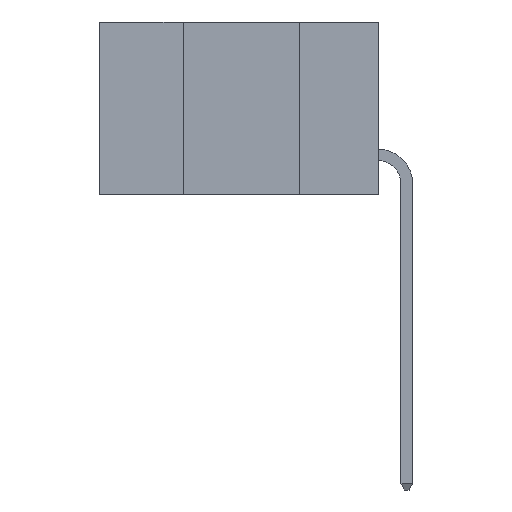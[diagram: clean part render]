
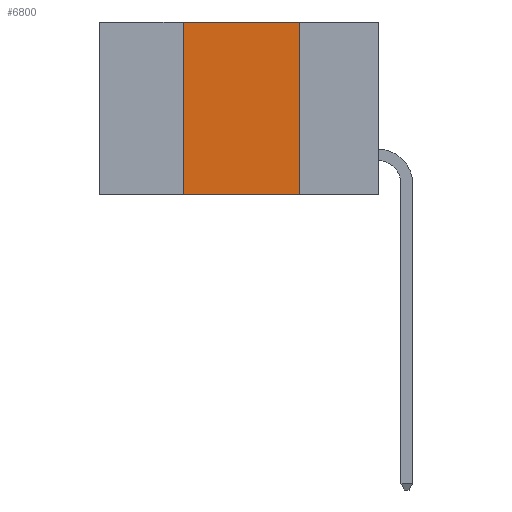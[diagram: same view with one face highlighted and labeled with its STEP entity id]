
A CAD part, left-side view. The second image highlights one B-rep face of the part: STEP entity #6800.
In plain terms, the highlighted planar face has unit normal (-1, 0, 0).
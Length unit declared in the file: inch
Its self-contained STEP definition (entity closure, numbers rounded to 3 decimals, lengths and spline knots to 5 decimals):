
#196 = LINE ( 'NONE', #5442, #4242 ) ;
#458 = CARTESIAN_POINT ( 'NONE',  ( 0., 0.6, -0.37 ) ) ;
#465 = CARTESIAN_POINT ( 'NONE',  ( 0., 0.42, -0.37 ) ) ;
#785 = CARTESIAN_POINT ( 'NONE',  ( 0., 0.17, -0.37 ) ) ;
#815 = EDGE_CURVE ( 'NONE', #5979, #6418, #4094, .T. ) ;
#880 = DIRECTION ( 'NONE',  ( 0., 0., -1. ) ) ;
#1025 = ORIENTED_EDGE ( 'NONE', *, *, #815, .T. ) ;
#1247 = DIRECTION ( 'NONE',  ( 0., -1., 0. ) ) ;
#1841 = VECTOR ( 'NONE', #7947, 39.37008 ) ;
#2918 = VERTEX_POINT ( 'NONE', #10349 ) ;
#3309 = LINE ( 'NONE', #8675, #5537 ) ;
#3411 = PLANE ( 'NONE',  #8020 ) ;
#3537 = VECTOR ( 'NONE', #880, 39.37008 ) ;
#3877 = EDGE_LOOP ( 'NONE', ( #5787, #9614, #7623, #1025 ) ) ;
#3914 = EDGE_CURVE ( 'NONE', #2918, #6418, #9583, .T. ) ;
#4094 = LINE ( 'NONE', #458, #1841 ) ;
#4242 = VECTOR ( 'NONE', #1247, 39.37008 ) ;
#4587 = CARTESIAN_POINT ( 'NONE',  ( 0., 0.42, 0. ) ) ;
#5096 = DIRECTION ( 'NONE',  ( 0., 0., -1. ) ) ;
#5289 = FACE_OUTER_BOUND ( 'NONE', #3877, .T. ) ;
#5442 = CARTESIAN_POINT ( 'NONE',  ( 0., 0.6, 0. ) ) ;
#5537 = VECTOR ( 'NONE', #9421, 39.37008 ) ;
#5787 = ORIENTED_EDGE ( 'NONE', *, *, #3914, .F. ) ;
#5979 = VERTEX_POINT ( 'NONE', #465 ) ;
#6262 = CARTESIAN_POINT ( 'NONE',  ( 0., 0.17, -0.37 ) ) ;
#6418 = VERTEX_POINT ( 'NONE', #6262 ) ;
#6800 = ADVANCED_FACE ( 'NONE', ( #5289 ), #3411, .F. ) ;
#7063 = VERTEX_POINT ( 'NONE', #4587 ) ;
#7171 = EDGE_CURVE ( 'NONE', #5979, #7063, #3309, .T. ) ;
#7623 = ORIENTED_EDGE ( 'NONE', *, *, #7171, .F. ) ;
#7688 = EDGE_CURVE ( 'NONE', #7063, #2918, #196, .T. ) ;
#7947 = DIRECTION ( 'NONE',  ( 0., -1., 0. ) ) ;
#8020 = AXIS2_PLACEMENT_3D ( 'NONE', #8959, #9730, #5096 ) ;
#8675 = CARTESIAN_POINT ( 'NONE',  ( 0., 0.42, -0.37 ) ) ;
#8959 = CARTESIAN_POINT ( 'NONE',  ( 0., 0.6, 0. ) ) ;
#9421 = DIRECTION ( 'NONE',  ( 0., 0., 1. ) ) ;
#9583 = LINE ( 'NONE', #785, #3537 ) ;
#9614 = ORIENTED_EDGE ( 'NONE', *, *, #7688, .F. ) ;
#9730 = DIRECTION ( 'NONE',  ( 1., 0., 0. ) ) ;
#10349 = CARTESIAN_POINT ( 'NONE',  ( 0., 0.17, 0. ) ) ;
